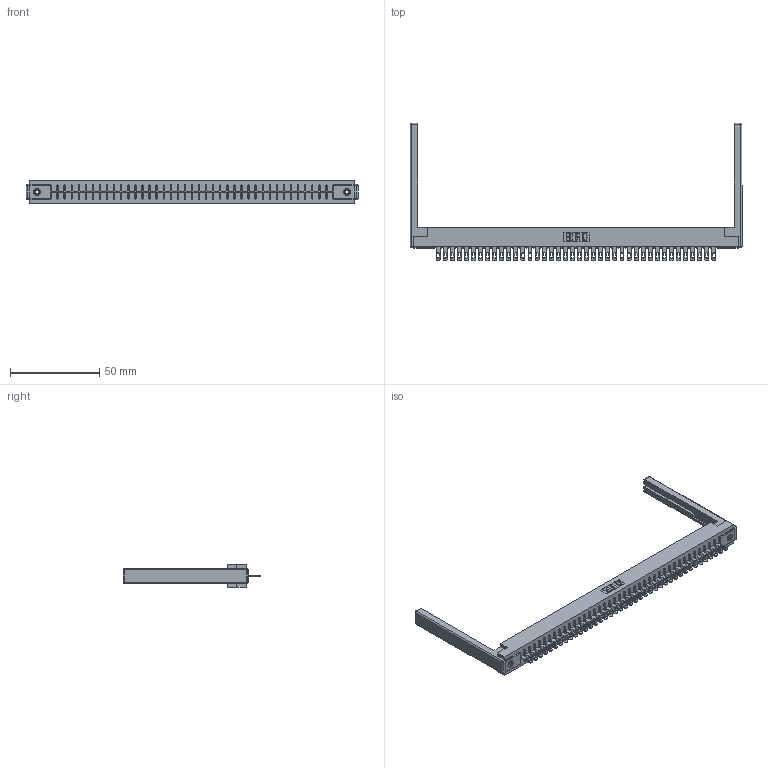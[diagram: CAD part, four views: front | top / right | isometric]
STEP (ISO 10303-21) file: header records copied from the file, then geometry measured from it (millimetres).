
FILE_DESCRIPTION (( 'STEP AP203' ), '1' );
FILE_NAME ('356-040-500-168.STEP', '2018-08-01T22:31:50', ( '' ), ( '' ), 'SwSTEP 2.0', 'SolidWorks 2016', '' );
FILE_SCHEMA (( 'CONFIG_CONTROL_DESIGN' ));
Length unit declared in the file: inch
Products named in the file (5): 306 Part_.156 Dia; 306-290-001_100; 345-250-001_345-250-001-102; 307-220-068; 356-040-500-168
Assembly tree (45 placements, depth 2):
  356-040-500-168
    306 Part_.156 Dia
    306-290-001_100  x40
    345-250-001_345-250-001-102  x2
    307-220-068  x2
Bounding box: 185.93 x 77.17 x 12.7 mm (x, y, z)
Volume: 25033.5 mm3; surface area: 25962.5 mm2
Topology: 45 solids, 45 shells, 3310 faces, 9306 edges, 5968 vertices
Faces by surface type: plane 2156, cylinder 970, sphere 168, cone 12, torus 4
Entity records: 40484 total; most frequent: CARTESIAN_POINT 6764, ORIENTED_EDGE 6698, DIRECTION 6683, EDGE_CURVE 3349, LINE 2613, VECTOR 2613, VERTEX_POINT 2116, AXIS2_PLACEMENT_3D 2035
